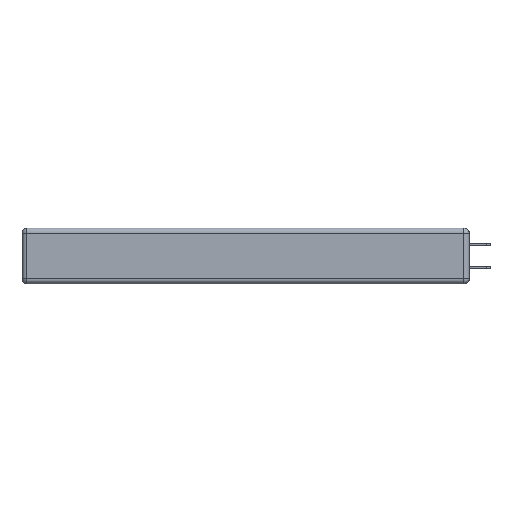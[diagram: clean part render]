
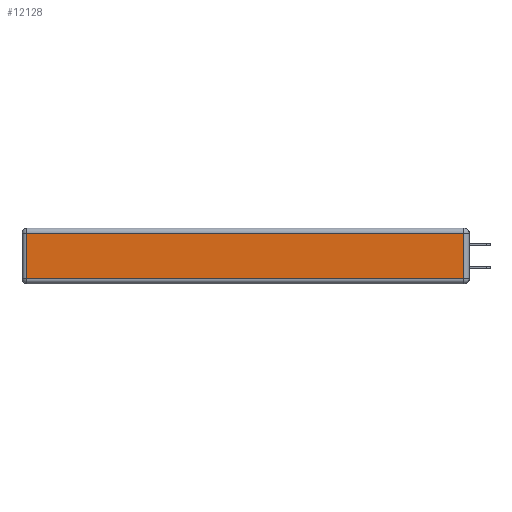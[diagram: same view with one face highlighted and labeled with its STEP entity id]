
A CAD part, left-side view. The second image highlights one B-rep face of the part: STEP entity #12128.
In plain terms, the highlighted planar face has unit normal (-1, 0, 0).
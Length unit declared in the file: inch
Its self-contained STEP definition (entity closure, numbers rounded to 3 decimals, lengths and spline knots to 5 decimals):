
#332 = CARTESIAN_POINT ( 'NONE',  ( 0., 0.03, -0.343 ) ) ;
#1521 = LINE ( 'NONE', #9557, #10416 ) ;
#2105 = EDGE_CURVE ( 'NONE', #13582, #5958, #1521, .T. ) ;
#2204 = ORIENTED_EDGE ( 'NONE', *, *, #11943, .T. ) ;
#2291 = DIRECTION ( 'NONE',  ( 0., 0., -1. ) ) ;
#2710 = VECTOR ( 'NONE', #12316, 39.37008 ) ;
#3913 = AXIS2_PLACEMENT_3D ( 'NONE', #14645, #13450, #8538 ) ;
#3981 = DIRECTION ( 'NONE',  ( 0., 0., 1. ) ) ;
#4058 = CARTESIAN_POINT ( 'NONE',  ( 0., 0.03, -0.03 ) ) ;
#4060 = VECTOR ( 'NONE', #2291, 39.37008 ) ;
#4522 = VECTOR ( 'NONE', #3981, 39.37008 ) ;
#4957 = CARTESIAN_POINT ( 'NONE',  ( 0., 2.72, -0.313 ) ) ;
#5501 = EDGE_LOOP ( 'NONE', ( #10258, #9348, #15401, #2204 ) ) ;
#5958 = VERTEX_POINT ( 'NONE', #8753 ) ;
#6904 = EDGE_CURVE ( 'NONE', #5958, #8964, #9730, .T. ) ;
#7569 = FACE_OUTER_BOUND ( 'NONE', #5501, .T. ) ;
#8012 = CARTESIAN_POINT ( 'NONE',  ( 0., 2.72, -0.343 ) ) ;
#8538 = DIRECTION ( 'NONE',  ( 0., 0., 1. ) ) ;
#8753 = CARTESIAN_POINT ( 'NONE',  ( 0., 0.03, -0.313 ) ) ;
#8863 = CARTESIAN_POINT ( 'NONE',  ( 0., 2.72, -0.03 ) ) ;
#8964 = VERTEX_POINT ( 'NONE', #4058 ) ;
#9235 = DIRECTION ( 'NONE',  ( 0., -1., 0. ) ) ;
#9348 = ORIENTED_EDGE ( 'NONE', *, *, #6904, .T. ) ;
#9557 = CARTESIAN_POINT ( 'NONE',  ( 0., 0., -0.313 ) ) ;
#9613 = LINE ( 'NONE', #8012, #4060 ) ;
#9730 = LINE ( 'NONE', #332, #4522 ) ;
#9812 = PLANE ( 'NONE',  #3913 ) ;
#9875 = CARTESIAN_POINT ( 'NONE',  ( 0., 2.75, -0.03 ) ) ;
#10258 = ORIENTED_EDGE ( 'NONE', *, *, #2105, .T. ) ;
#10416 = VECTOR ( 'NONE', #9235, 39.37008 ) ;
#11943 = EDGE_CURVE ( 'NONE', #14793, #13582, #9613, .T. ) ;
#12128 = ADVANCED_FACE ( 'NONE', ( #7569 ), #9812, .T. ) ;
#12316 = DIRECTION ( 'NONE',  ( 0., 1., 0. ) ) ;
#12930 = LINE ( 'NONE', #9875, #2710 ) ;
#13405 = EDGE_CURVE ( 'NONE', #8964, #14793, #12930, .T. ) ;
#13450 = DIRECTION ( 'NONE',  ( -1., 0., 0. ) ) ;
#13582 = VERTEX_POINT ( 'NONE', #4957 ) ;
#14645 = CARTESIAN_POINT ( 'NONE',  ( 0., 0., -0.343 ) ) ;
#14793 = VERTEX_POINT ( 'NONE', #8863 ) ;
#15401 = ORIENTED_EDGE ( 'NONE', *, *, #13405, .T. ) ;
